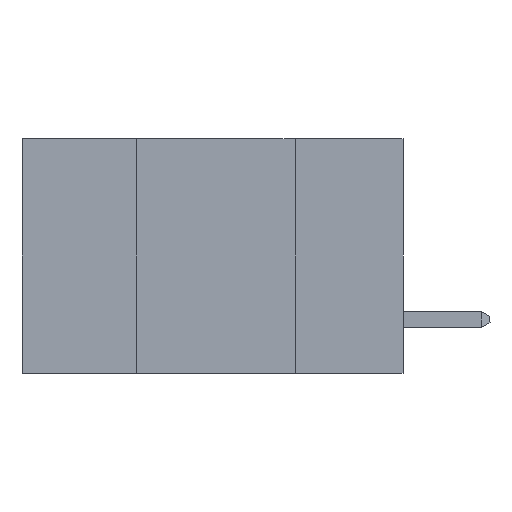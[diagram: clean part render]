
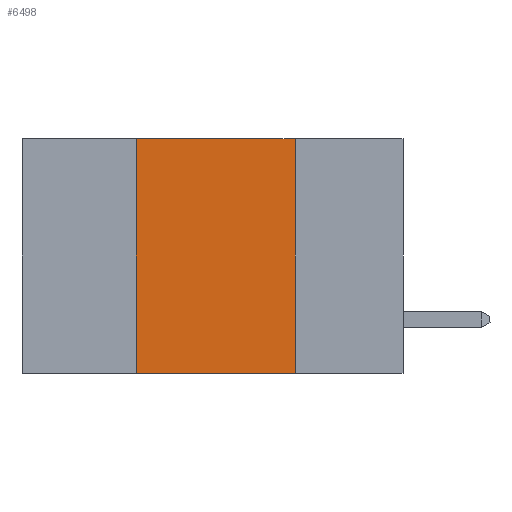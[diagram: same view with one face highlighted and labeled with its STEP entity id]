
A CAD part, left-side view. The second image highlights one B-rep face of the part: STEP entity #6498.
In plain terms, the highlighted planar face has unit normal (-1, 0, 0).
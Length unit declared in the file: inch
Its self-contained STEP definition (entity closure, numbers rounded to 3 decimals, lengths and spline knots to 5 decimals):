
#610 = VECTOR ( 'NONE', #17698, 39.37008 ) ;
#1887 = CARTESIAN_POINT ( 'NONE',  ( 0., 0.42, 0. ) ) ;
#1964 = DIRECTION ( 'NONE',  ( 0., 0., 1. ) ) ;
#2743 = CARTESIAN_POINT ( 'NONE',  ( 0., 0.6, 0. ) ) ;
#3120 = DIRECTION ( 'NONE',  ( 0., 0., -1. ) ) ;
#3318 = DIRECTION ( 'NONE',  ( 1., 0., 0. ) ) ;
#3789 = EDGE_CURVE ( 'NONE', #8188, #20122, #7846, .T. ) ;
#4100 = ORIENTED_EDGE ( 'NONE', *, *, #9922, .F. ) ;
#4339 = VERTEX_POINT ( 'NONE', #9013 ) ;
#4410 = DIRECTION ( 'NONE',  ( 0., -1., 0. ) ) ;
#4488 = AXIS2_PLACEMENT_3D ( 'NONE', #13397, #3318, #15130 ) ;
#5146 = ORIENTED_EDGE ( 'NONE', *, *, #16258, .T. ) ;
#5837 = CARTESIAN_POINT ( 'NONE',  ( 0., 0.6, -0.37 ) ) ;
#6333 = CARTESIAN_POINT ( 'NONE',  ( 0., 0.42, 0. ) ) ;
#6498 = ADVANCED_FACE ( 'NONE', ( #20371 ), #11671, .F. ) ;
#6830 = EDGE_LOOP ( 'NONE', ( #19206, #4100, #20507, #5146 ) ) ;
#7846 = LINE ( 'NONE', #1887, #12390 ) ;
#8188 = VERTEX_POINT ( 'NONE', #9668 ) ;
#9013 = CARTESIAN_POINT ( 'NONE',  ( 0., 0.17, -0.37 ) ) ;
#9668 = CARTESIAN_POINT ( 'NONE',  ( 0., 0.42, -0.37 ) ) ;
#9922 = EDGE_CURVE ( 'NONE', #20122, #21843, #13029, .T. ) ;
#11671 = PLANE ( 'NONE',  #4488 ) ;
#12390 = VECTOR ( 'NONE', #1964, 39.37008 ) ;
#13029 = LINE ( 'NONE', #2743, #17021 ) ;
#13194 = CARTESIAN_POINT ( 'NONE',  ( 0., 0.17, 0. ) ) ;
#13397 = CARTESIAN_POINT ( 'NONE',  ( 0., 0.6, 0. ) ) ;
#13635 = LINE ( 'NONE', #13194, #17615 ) ;
#14125 = LINE ( 'NONE', #5837, #610 ) ;
#15130 = DIRECTION ( 'NONE',  ( 0., 0., -1. ) ) ;
#16258 = EDGE_CURVE ( 'NONE', #8188, #4339, #14125, .T. ) ;
#16450 = CARTESIAN_POINT ( 'NONE',  ( 0., 0.17, 0. ) ) ;
#17021 = VECTOR ( 'NONE', #4410, 39.37008 ) ;
#17615 = VECTOR ( 'NONE', #3120, 39.37008 ) ;
#17698 = DIRECTION ( 'NONE',  ( 0., -1., 0. ) ) ;
#19206 = ORIENTED_EDGE ( 'NONE', *, *, #21284, .F. ) ;
#20122 = VERTEX_POINT ( 'NONE', #6333 ) ;
#20371 = FACE_OUTER_BOUND ( 'NONE', #6830, .T. ) ;
#20507 = ORIENTED_EDGE ( 'NONE', *, *, #3789, .F. ) ;
#21284 = EDGE_CURVE ( 'NONE', #21843, #4339, #13635, .T. ) ;
#21843 = VERTEX_POINT ( 'NONE', #16450 ) ;
